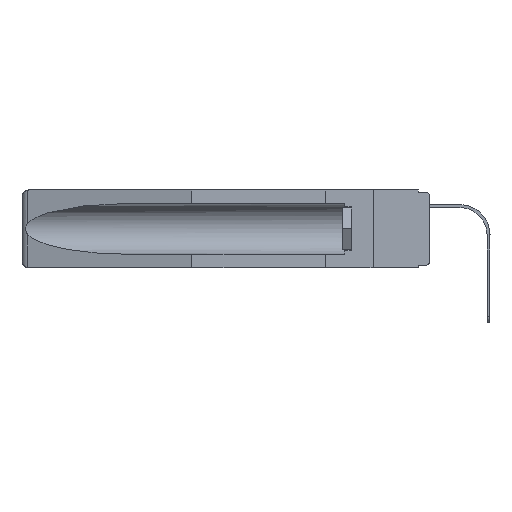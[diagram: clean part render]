
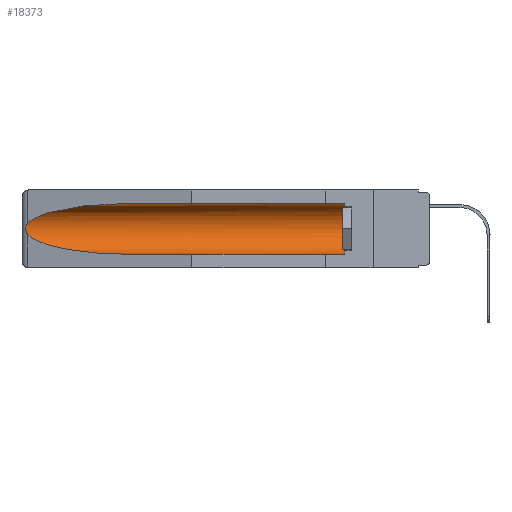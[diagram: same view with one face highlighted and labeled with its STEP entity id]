
A CAD part, left-side view. The second image highlights one B-rep face of the part: STEP entity #18373.
In plain terms, the highlighted cylindrical face has radius 2.857 mm (diameter 5.715 mm), a partial arc.
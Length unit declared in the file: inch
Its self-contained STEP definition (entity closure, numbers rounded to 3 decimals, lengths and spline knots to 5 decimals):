
#16 = ORIENTED_EDGE ( 'NONE', *, *, #11631, .T. ) ;
#901 = DIRECTION ( 'NONE',  ( 0., 0., 1. ) ) ;
#1084 = FACE_OUTER_BOUND ( 'NONE', #10130, .T. ) ;
#2318 = CARTESIAN_POINT ( 'NONE',  ( 0.2675, 1.53308, -0.17534 ) ) ;
#2321 = CARTESIAN_POINT ( 'NONE',  ( 0.25451, 1.48313, -0.24835 ) ) ;
#2946 = ORIENTED_EDGE ( 'NONE', *, *, #11474, .T. ) ;
#3066 = EDGE_CURVE ( 'NONE', #3352, #15494, #12217, .T. ) ;
#3352 = VERTEX_POINT ( 'NONE', #10602 ) ;
#3727 = VECTOR ( 'NONE', #14593, 39.37008 ) ;
#3740 = CARTESIAN_POINT ( 'NONE',  ( 0.26597, 1.52961, -0.15275 ) ) ;
#3743 = CARTESIAN_POINT ( 'NONE',  ( 0.155, 1.07973, -0.284 ) ) ;
#3850 = CARTESIAN_POINT ( 'NONE',  ( 0.155, 1.07973, -0.059 ) ) ;
#4123 = DIRECTION ( 'NONE',  ( 0., 0., 1. ) ) ;
#4709 = CIRCLE ( 'NONE', #12622, 0.1125 ) ;
#4821 = EDGE_CURVE ( 'NONE', #15494, #8229, #13418, .T. ) ;
#6113 = VERTEX_POINT ( 'NONE', #3850 ) ;
#6412 = CARTESIAN_POINT ( 'NONE',  ( 0.155, -0.30754, -0.059 ) ) ;
#6974 = CYLINDRICAL_SURFACE ( 'NONE', #7832, 0.1125 ) ;
#7173 = CARTESIAN_POINT ( 'NONE',  ( 0.155, -0.30754, -0.1715 ) ) ;
#7224 = VERTEX_POINT ( 'NONE', #13462 ) ;
#7717 = DIRECTION ( 'NONE',  ( 0., 1., 0. ) ) ;
#7832 = AXIS2_PLACEMENT_3D ( 'NONE', #7173, #17123, #4123 ) ;
#8137 = CARTESIAN_POINT ( 'NONE',  ( 0.2673, 1.53269, -0.17917 ) ) ;
#8225 = CARTESIAN_POINT ( 'NONE',  ( 0.26655, 1.53094, -0.18657 ) ) ;
#8229 = VERTEX_POINT ( 'NONE', #16694 ) ;
#8517 = ORIENTED_EDGE ( 'NONE', *, *, #9106, .T. ) ;
#9049 = LINE ( 'NONE', #16332, #17427 ) ;
#9106 = EDGE_CURVE ( 'NONE', #9120, #7224, #4709, .T. ) ;
#9120 = VERTEX_POINT ( 'NONE', #11207 ) ;
#9277 = LINE ( 'NONE', #6412, #3727 ) ;
#9301 = ORIENTED_EDGE ( 'NONE', *, *, #3066, .T. ) ;
#9544 = CARTESIAN_POINT ( 'NONE',  ( 0.2673, 1.5327, -0.16383 ) ) ;
#10130 = EDGE_LOOP ( 'NONE', ( #2946, #9301, #12063, #10312, #8517, #16 ) ) ;
#10312 = ORIENTED_EDGE ( 'NONE', *, *, #15467, .F. ) ;
#10315 =( BOUNDED_CURVE ( )  B_SPLINE_CURVE ( 3, ( #14221, #17071, #18410, #11238 ),
 .UNSPECIFIED., .F., .F. ) 
 B_SPLINE_CURVE_WITH_KNOTS ( ( 4, 4 ),
 ( 4.71239, 6.08839 ),
 .UNSPECIFIED. ) 
 CURVE ( )  GEOMETRIC_REPRESENTATION_ITEM ( )  RATIONAL_B_SPLINE_CURVE ( ( 1., 0.848, 0.848, 1. ) ) 
 REPRESENTATION_ITEM ( '' )  );
#10602 = CARTESIAN_POINT ( 'NONE',  ( 0.26537, 1.52718, -0.14972 ) ) ;
#11087 = CARTESIAN_POINT ( 'NONE',  ( 0.26537, 1.52718, -0.19328 ) ) ;
#11207 = CARTESIAN_POINT ( 'NONE',  ( 0.155, 0.126, -0.284 ) ) ;
#11238 = CARTESIAN_POINT ( 'NONE',  ( 0.26537, 1.52718, -0.14972 ) ) ;
#11474 = EDGE_CURVE ( 'NONE', #6113, #3352, #10315, .T. ) ;
#11631 = EDGE_CURVE ( 'NONE', #7224, #6113, #9277, .T. ) ;
#11889 = CARTESIAN_POINT ( 'NONE',  ( 0.26537, 1.52718, -0.19328 ) ) ;
#12063 = ORIENTED_EDGE ( 'NONE', *, *, #4821, .T. ) ;
#12217 = B_SPLINE_CURVE_WITH_KNOTS ( 'NONE', 3,
 ( #12389, #3740, #17966, #9544, #15302, #2318, #8137, #8225, #18243, #11087 ),
 .UNSPECIFIED., .F., .F.,
 ( 4, 2, 2, 2, 4 ),
 ( 0., 0.00029, 0.00058, 0.00087, 0.00117 ),
 .UNSPECIFIED. ) ;
#12389 = CARTESIAN_POINT ( 'NONE',  ( 0.26537, 1.52718, -0.14972 ) ) ;
#12622 = AXIS2_PLACEMENT_3D ( 'NONE', #16863, #15326, #901 ) ;
#13418 =( BOUNDED_CURVE ( )  B_SPLINE_CURVE ( 3, ( #15495, #2321, #13986, #3743 ),
 .UNSPECIFIED., .F., .F. ) 
 B_SPLINE_CURVE_WITH_KNOTS ( ( 4, 4 ),
 ( 0.1948, 1.5708 ),
 .UNSPECIFIED. ) 
 CURVE ( )  GEOMETRIC_REPRESENTATION_ITEM ( )  RATIONAL_B_SPLINE_CURVE ( ( 1., 0.848, 0.848, 1. ) ) 
 REPRESENTATION_ITEM ( '' )  );
#13462 = CARTESIAN_POINT ( 'NONE',  ( 0.155, 0.126, -0.059 ) ) ;
#13986 = CARTESIAN_POINT ( 'NONE',  ( 0.21114, 1.30732, -0.284 ) ) ;
#14221 = CARTESIAN_POINT ( 'NONE',  ( 0.155, 1.07973, -0.059 ) ) ;
#14593 = DIRECTION ( 'NONE',  ( 0., 1., 0. ) ) ;
#15302 = CARTESIAN_POINT ( 'NONE',  ( 0.2675, 1.53308, -0.16763 ) ) ;
#15326 = DIRECTION ( 'NONE',  ( 0., -1., 0. ) ) ;
#15467 = EDGE_CURVE ( 'NONE', #9120, #8229, #9049, .T. ) ;
#15494 = VERTEX_POINT ( 'NONE', #11889 ) ;
#15495 = CARTESIAN_POINT ( 'NONE',  ( 0.26537, 1.52718, -0.19328 ) ) ;
#16332 = CARTESIAN_POINT ( 'NONE',  ( 0.155, -0.30754, -0.284 ) ) ;
#16694 = CARTESIAN_POINT ( 'NONE',  ( 0.155, 1.07973, -0.284 ) ) ;
#16863 = CARTESIAN_POINT ( 'NONE',  ( 0.155, 0.126, -0.1715 ) ) ;
#17071 = CARTESIAN_POINT ( 'NONE',  ( 0.21114, 1.30732, -0.059 ) ) ;
#17123 = DIRECTION ( 'NONE',  ( 0., 1., 0. ) ) ;
#17427 = VECTOR ( 'NONE', #7717, 39.37008 ) ;
#17966 = CARTESIAN_POINT ( 'NONE',  ( 0.26654, 1.53092, -0.15636 ) ) ;
#18243 = CARTESIAN_POINT ( 'NONE',  ( 0.26597, 1.5296, -0.19026 ) ) ;
#18373 = ADVANCED_FACE ( 'NONE', ( #1084 ), #6974, .F. ) ;
#18410 = CARTESIAN_POINT ( 'NONE',  ( 0.25451, 1.48313, -0.09465 ) ) ;
